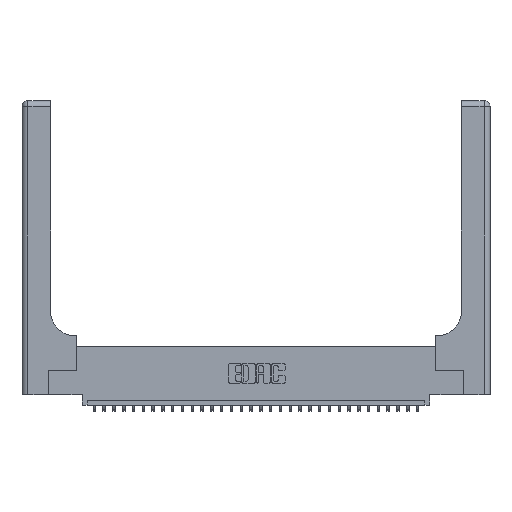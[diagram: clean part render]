
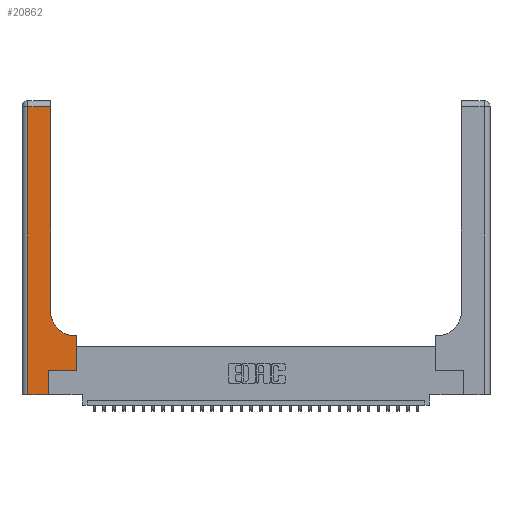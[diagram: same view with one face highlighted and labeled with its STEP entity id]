
A CAD part, top view. The second image highlights one B-rep face of the part: STEP entity #20862.
In plain terms, the highlighted planar face has unit normal (0, 0, 1).
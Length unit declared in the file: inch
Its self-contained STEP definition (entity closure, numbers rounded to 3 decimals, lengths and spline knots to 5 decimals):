
#109 = VECTOR ( 'NONE', #11961, 39.37008 ) ;
#407 = EDGE_CURVE ( 'NONE', #13156, #8498, #5771, .T. ) ;
#428 = CARTESIAN_POINT ( 'NONE',  ( 0.5585, 0.25, 0.37 ) ) ;
#1544 = CARTESIAN_POINT ( 'NONE',  ( 0.5585, 0.25, 0.37 ) ) ;
#3028 = ORIENTED_EDGE ( 'NONE', *, *, #407, .T. ) ;
#3160 = VERTEX_POINT ( 'NONE', #1544 ) ;
#3170 = LINE ( 'NONE', #28777, #22956 ) ;
#4792 = LINE ( 'NONE', #29367, #109 ) ;
#5600 = CARTESIAN_POINT ( 'NONE',  ( 0.269, 0., 0.37 ) ) ;
#5663 = ORIENTED_EDGE ( 'NONE', *, *, #8913, .T. ) ;
#5771 = LINE ( 'NONE', #20961, #11608 ) ;
#6135 = VECTOR ( 'NONE', #20371, 39.37008 ) ;
#6277 = DIRECTION ( 'NONE',  ( 0., 1., 0. ) ) ;
#6328 = CARTESIAN_POINT ( 'NONE',  ( 0.2915, 2.94, 0.37 ) ) ;
#6669 = ORIENTED_EDGE ( 'NONE', *, *, #21158, .T. ) ;
#7031 = ORIENTED_EDGE ( 'NONE', *, *, #21505, .T. ) ;
#7218 = CARTESIAN_POINT ( 'NONE',  ( 0.2915, 0.6, 0.37 ) ) ;
#7884 = DIRECTION ( 'NONE',  ( 0., 1., 0. ) ) ;
#8498 = VERTEX_POINT ( 'NONE', #5600 ) ;
#8647 = PLANE ( 'NONE',  #12484 ) ;
#8760 = CARTESIAN_POINT ( 'NONE',  ( 0., 3., 0.37 ) ) ;
#8913 = EDGE_CURVE ( 'NONE', #12459, #25844, #31527, .T. ) ;
#9073 = CARTESIAN_POINT ( 'NONE',  ( 0., 2.94, 0.37 ) ) ;
#9690 = DIRECTION ( 'NONE',  ( -1., 0., 0. ) ) ;
#10074 = CARTESIAN_POINT ( 'NONE',  ( 0.5415, 0.85, 0.37 ) ) ;
#10383 = LINE ( 'NONE', #428, #6135 ) ;
#10875 = CARTESIAN_POINT ( 'NONE',  ( 0.2915, 0.85, 0.37 ) ) ;
#11027 = DIRECTION ( 'NONE',  ( -1., 0., 0. ) ) ;
#11608 = VECTOR ( 'NONE', #13509, 39.37008 ) ;
#11961 = DIRECTION ( 'NONE',  ( 0., -1., 0. ) ) ;
#12197 = VECTOR ( 'NONE', #6277, 39.37008 ) ;
#12370 = DIRECTION ( 'NONE',  ( 1., 0., 0. ) ) ;
#12459 = VERTEX_POINT ( 'NONE', #28051 ) ;
#12484 = AXIS2_PLACEMENT_3D ( 'NONE', #8760, #28576, #11027 ) ;
#12565 = LINE ( 'NONE', #7218, #28877 ) ;
#12752 = CARTESIAN_POINT ( 'NONE',  ( 0.269, 0., 0.37 ) ) ;
#13156 = VERTEX_POINT ( 'NONE', #29663 ) ;
#13509 = DIRECTION ( 'NONE',  ( 1., 0., 0. ) ) ;
#14037 = DIRECTION ( 'NONE',  ( -1., 0., 0. ) ) ;
#15112 = CARTESIAN_POINT ( 'NONE',  ( 0.5585, 0.6, 0.37 ) ) ;
#15229 = EDGE_CURVE ( 'NONE', #25844, #31936, #23452, .T. ) ;
#15881 = EDGE_CURVE ( 'NONE', #3160, #24972, #10383, .T. ) ;
#15974 = LINE ( 'NONE', #12752, #26034 ) ;
#16569 = EDGE_CURVE ( 'NONE', #8498, #28736, #15974, .T. ) ;
#17244 = FACE_OUTER_BOUND ( 'NONE', #25416, .T. ) ;
#17652 = DIRECTION ( 'NONE',  ( 0., 0., -1. ) ) ;
#17997 = ORIENTED_EDGE ( 'NONE', *, *, #30151, .T. ) ;
#18348 = CARTESIAN_POINT ( 'NONE',  ( 0.269, 0.25, 0.37 ) ) ;
#19958 = ORIENTED_EDGE ( 'NONE', *, *, #16569, .T. ) ;
#20371 = DIRECTION ( 'NONE',  ( 0., 1., 0. ) ) ;
#20862 = ADVANCED_FACE ( 'NONE', ( #17244 ), #8647, .F. ) ;
#20961 = CARTESIAN_POINT ( 'NONE',  ( 0., 0., 0.37 ) ) ;
#21158 = EDGE_CURVE ( 'NONE', #24972, #12459, #12565, .T. ) ;
#21505 = EDGE_CURVE ( 'NONE', #31669, #13156, #4792, .T. ) ;
#22575 = AXIS2_PLACEMENT_3D ( 'NONE', #10074, #17652, #12370 ) ;
#22956 = VECTOR ( 'NONE', #26486, 39.37008 ) ;
#23452 = LINE ( 'NONE', #26184, #12197 ) ;
#24223 = LINE ( 'NONE', #9073, #26132 ) ;
#24234 = ORIENTED_EDGE ( 'NONE', *, *, #15881, .T. ) ;
#24814 = ORIENTED_EDGE ( 'NONE', *, *, #15229, .T. ) ;
#24972 = VERTEX_POINT ( 'NONE', #15112 ) ;
#25416 = EDGE_LOOP ( 'NONE', ( #24814, #30207, #7031, #3028, #19958, #17997, #24234, #6669, #5663 ) ) ;
#25844 = VERTEX_POINT ( 'NONE', #10875 ) ;
#26034 = VECTOR ( 'NONE', #7884, 39.37008 ) ;
#26132 = VECTOR ( 'NONE', #14037, 39.37008 ) ;
#26184 = CARTESIAN_POINT ( 'NONE',  ( 0.2915, 3., 0.37 ) ) ;
#26486 = DIRECTION ( 'NONE',  ( 1., 0., 0. ) ) ;
#27252 = EDGE_CURVE ( 'NONE', #31936, #31669, #24223, .T. ) ;
#28051 = CARTESIAN_POINT ( 'NONE',  ( 0.5415, 0.6, 0.37 ) ) ;
#28283 = CARTESIAN_POINT ( 'NONE',  ( 0.06, 2.94, 0.37 ) ) ;
#28576 = DIRECTION ( 'NONE',  ( 0., 0., -1. ) ) ;
#28736 = VERTEX_POINT ( 'NONE', #18348 ) ;
#28777 = CARTESIAN_POINT ( 'NONE',  ( 0.269, 0.25, 0.37 ) ) ;
#28877 = VECTOR ( 'NONE', #9690, 39.37008 ) ;
#29367 = CARTESIAN_POINT ( 'NONE',  ( 0.06, 3., 0.37 ) ) ;
#29663 = CARTESIAN_POINT ( 'NONE',  ( 0.06, 0., 0.37 ) ) ;
#30151 = EDGE_CURVE ( 'NONE', #28736, #3160, #3170, .T. ) ;
#30207 = ORIENTED_EDGE ( 'NONE', *, *, #27252, .T. ) ;
#31527 = CIRCLE ( 'NONE', #22575, 0.25 ) ;
#31669 = VERTEX_POINT ( 'NONE', #28283 ) ;
#31936 = VERTEX_POINT ( 'NONE', #6328 ) ;
